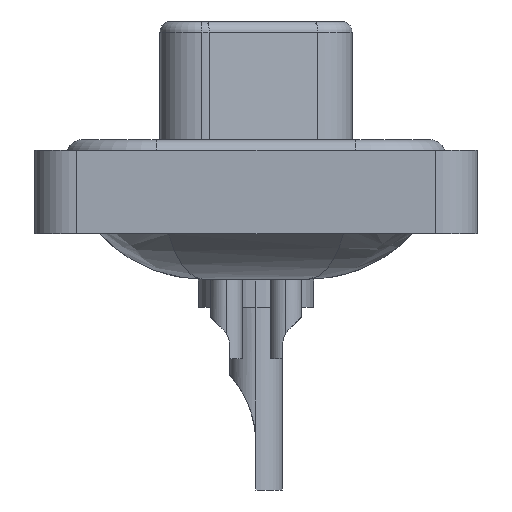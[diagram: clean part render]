
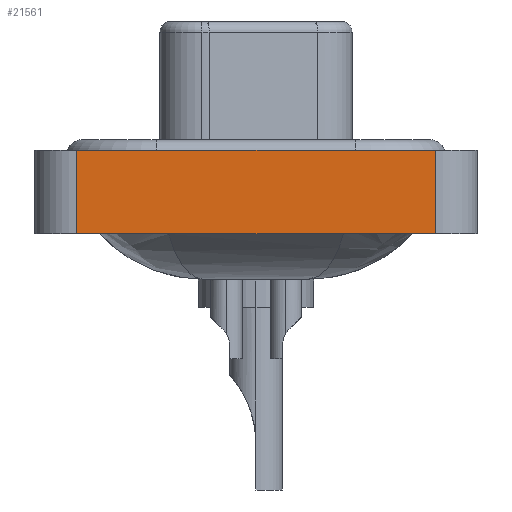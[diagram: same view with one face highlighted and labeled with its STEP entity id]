
A CAD part, left-side view. The second image highlights one B-rep face of the part: STEP entity #21561.
In plain terms, the highlighted planar face has unit normal (-1, 0, 0).
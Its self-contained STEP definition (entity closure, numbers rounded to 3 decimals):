
#177 = CARTESIAN_POINT ( 'NONE',  ( -7.35, -8.55, 0.4 ) ) ;
#683 = EDGE_CURVE ( 'NONE', #12392, #6676, #11753, .T. ) ;
#2019 = LINE ( 'NONE', #9672, #23239 ) ;
#2323 = AXIS2_PLACEMENT_3D ( 'NONE', #19322, #20965, #2668 ) ;
#2466 = ORIENTED_EDGE ( 'NONE', *, *, #23660, .T. ) ;
#2668 = DIRECTION ( 'NONE',  ( 0., 0., 1. ) ) ;
#2730 = EDGE_CURVE ( 'NONE', #12392, #24686, #2019, .T. ) ;
#3263 = EDGE_LOOP ( 'NONE', ( #2466, #13537, #5304, #9360 ) ) ;
#3993 = CARTESIAN_POINT ( 'NONE',  ( -7.35, 8.55, -3.6 ) ) ;
#4055 = PLANE ( 'NONE',  #2323 ) ;
#4594 = CARTESIAN_POINT ( 'NONE',  ( -7.35, 8.55, -3.6 ) ) ;
#5304 = ORIENTED_EDGE ( 'NONE', *, *, #683, .F. ) ;
#5929 = FACE_OUTER_BOUND ( 'NONE', #3263, .T. ) ;
#6676 = VERTEX_POINT ( 'NONE', #7101 ) ;
#7000 = LINE ( 'NONE', #14752, #23067 ) ;
#7101 = CARTESIAN_POINT ( 'NONE',  ( -7.35, 8.55, 0.4 ) ) ;
#7573 = CARTESIAN_POINT ( 'NONE',  ( -7.35, -8.55, -3.6 ) ) ;
#9360 = ORIENTED_EDGE ( 'NONE', *, *, #2730, .T. ) ;
#9672 = CARTESIAN_POINT ( 'NONE',  ( -7.35, -8.55, -3.6 ) ) ;
#11071 = EDGE_CURVE ( 'NONE', #6676, #24422, #16423, .T. ) ;
#11582 = VECTOR ( 'NONE', #18189, 1000. ) ;
#11753 = LINE ( 'NONE', #3993, #18317 ) ;
#12392 = VERTEX_POINT ( 'NONE', #4594 ) ;
#12557 = CARTESIAN_POINT ( 'NONE',  ( -7.35, -8.55, 0.4 ) ) ;
#13537 = ORIENTED_EDGE ( 'NONE', *, *, #11071, .F. ) ;
#13871 = DIRECTION ( 'NONE',  ( 0., 0., 1. ) ) ;
#14752 = CARTESIAN_POINT ( 'NONE',  ( -7.35, -8.55, -3.6 ) ) ;
#16423 = LINE ( 'NONE', #12557, #11582 ) ;
#16614 = DIRECTION ( 'NONE',  ( 0., 0., 1. ) ) ;
#17528 = DIRECTION ( 'NONE',  ( 0., -1., 0. ) ) ;
#18189 = DIRECTION ( 'NONE',  ( 0., -1., 0. ) ) ;
#18317 = VECTOR ( 'NONE', #13871, 1000. ) ;
#19322 = CARTESIAN_POINT ( 'NONE',  ( -7.35, -8.55, -3.6 ) ) ;
#20965 = DIRECTION ( 'NONE',  ( -1., 0., 0. ) ) ;
#21561 = ADVANCED_FACE ( 'NONE', ( #5929 ), #4055, .T. ) ;
#23067 = VECTOR ( 'NONE', #16614, 1000. ) ;
#23239 = VECTOR ( 'NONE', #17528, 1000. ) ;
#23660 = EDGE_CURVE ( 'NONE', #24686, #24422, #7000, .T. ) ;
#24422 = VERTEX_POINT ( 'NONE', #177 ) ;
#24686 = VERTEX_POINT ( 'NONE', #7573 ) ;
